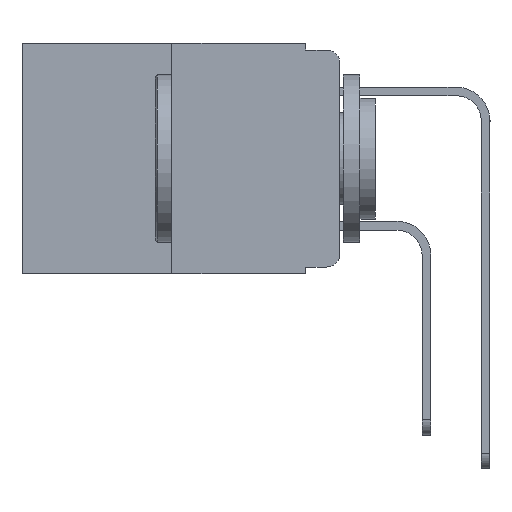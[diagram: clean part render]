
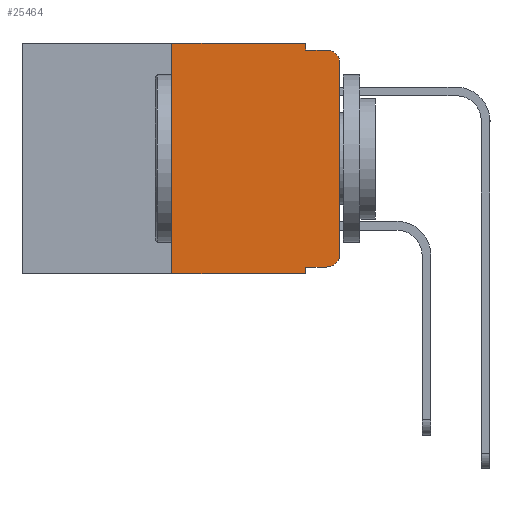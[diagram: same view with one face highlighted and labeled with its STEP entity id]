
A CAD part, left-side view. The second image highlights one B-rep face of the part: STEP entity #25464.
In plain terms, the highlighted planar face has unit normal (-1, 0, 0).
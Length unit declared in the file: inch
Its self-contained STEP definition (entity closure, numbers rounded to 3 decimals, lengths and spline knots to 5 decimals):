
#24 = ORIENTED_EDGE ( 'NONE', *, *, #26438, .T. ) ;
#459 = LINE ( 'NONE', #10308, #4694 ) ;
#638 = CARTESIAN_POINT ( 'NONE',  ( 0., 0.25, 0. ) ) ;
#872 = DIRECTION ( 'NONE',  ( -1., 0., 0. ) ) ;
#988 = CARTESIAN_POINT ( 'NONE',  ( 0., 0., -0.313 ) ) ;
#1020 = CARTESIAN_POINT ( 'NONE',  ( 0., 0.473, 0. ) ) ;
#1045 = VECTOR ( 'NONE', #23767, 39.37008 ) ;
#1234 = VERTEX_POINT ( 'NONE', #17863 ) ;
#1333 = EDGE_CURVE ( 'NONE', #17584, #11940, #21363, .T. ) ;
#1500 = VERTEX_POINT ( 'NONE', #988 ) ;
#1569 = ORIENTED_EDGE ( 'NONE', *, *, #6924, .F. ) ;
#1661 = ORIENTED_EDGE ( 'NONE', *, *, #5514, .F. ) ;
#1730 = DIRECTION ( 'NONE',  ( 0., 0., -1. ) ) ;
#3097 = DIRECTION ( 'NONE',  ( 0., 0., 1. ) ) ;
#3504 = CIRCLE ( 'NONE', #10316, 0.02 ) ;
#4107 = DIRECTION ( 'NONE',  ( 0., -1., 0. ) ) ;
#4131 = EDGE_CURVE ( 'NONE', #1234, #20670, #12058, .T. ) ;
#4135 = CARTESIAN_POINT ( 'NONE',  ( 0., 0.051, -0.01 ) ) ;
#4596 = ORIENTED_EDGE ( 'NONE', *, *, #8318, .T. ) ;
#4694 = VECTOR ( 'NONE', #23948, 39.37008 ) ;
#4937 = CARTESIAN_POINT ( 'NONE',  ( 0., 0., -0.03 ) ) ;
#5241 = CARTESIAN_POINT ( 'NONE',  ( 0., 0.25, 0. ) ) ;
#5342 = FACE_OUTER_BOUND ( 'NONE', #8882, .T. ) ;
#5514 = EDGE_CURVE ( 'NONE', #20888, #10586, #6510, .T. ) ;
#5902 = ORIENTED_EDGE ( 'NONE', *, *, #23820, .T. ) ;
#6167 = PLANE ( 'NONE',  #19599 ) ;
#6510 = LINE ( 'NONE', #13125, #22147 ) ;
#6924 = EDGE_CURVE ( 'NONE', #10586, #23219, #25503, .T. ) ;
#7121 = VERTEX_POINT ( 'NONE', #4937 ) ;
#7140 = DIRECTION ( 'NONE',  ( 0., -1., 0. ) ) ;
#8240 = DIRECTION ( 'NONE',  ( 0., 0., -1. ) ) ;
#8318 = EDGE_CURVE ( 'NONE', #7121, #23219, #20580, .T. ) ;
#8343 = VECTOR ( 'NONE', #18704, 39.37008 ) ;
#8415 = VECTOR ( 'NONE', #3097, 39.37008 ) ;
#8749 = LINE ( 'NONE', #1020, #24350 ) ;
#8882 = EDGE_LOOP ( 'NONE', ( #9433, #4596, #1569, #1661, #17804, #15344, #12168, #11025, #24, #5902 ) ) ;
#8999 = EDGE_CURVE ( 'NONE', #20670, #20888, #8749, .T. ) ;
#9433 = ORIENTED_EDGE ( 'NONE', *, *, #9685, .T. ) ;
#9613 = LINE ( 'NONE', #16665, #8343 ) ;
#9685 = EDGE_CURVE ( 'NONE', #1500, #7121, #13895, .T. ) ;
#9777 = CARTESIAN_POINT ( 'NONE',  ( 0., 0.02, -0.313 ) ) ;
#9812 = CARTESIAN_POINT ( 'NONE',  ( 0., 0.02, -0.01 ) ) ;
#9957 = CARTESIAN_POINT ( 'NONE',  ( 0., 0.051, -0.01 ) ) ;
#9986 = VECTOR ( 'NONE', #4107, 39.37008 ) ;
#10217 = CARTESIAN_POINT ( 'NONE',  ( 0., 0.473, 0. ) ) ;
#10308 = CARTESIAN_POINT ( 'NONE',  ( 0., 0.473, -0.343 ) ) ;
#10316 = AXIS2_PLACEMENT_3D ( 'NONE', #9777, #24016, #11842 ) ;
#10586 = VERTEX_POINT ( 'NONE', #9957 ) ;
#11000 = CARTESIAN_POINT ( 'NONE',  ( 0., 0.051, -0.333 ) ) ;
#11025 = ORIENTED_EDGE ( 'NONE', *, *, #1333, .F. ) ;
#11171 = DIRECTION ( 'NONE',  ( 0., 0., -1. ) ) ;
#11842 = DIRECTION ( 'NONE',  ( 0., 0., -1. ) ) ;
#11940 = VERTEX_POINT ( 'NONE', #12502 ) ;
#12058 = LINE ( 'NONE', #638, #1045 ) ;
#12168 = ORIENTED_EDGE ( 'NONE', *, *, #25477, .T. ) ;
#12502 = CARTESIAN_POINT ( 'NONE',  ( 0., 0.051, -0.343 ) ) ;
#13125 = CARTESIAN_POINT ( 'NONE',  ( 0., 0.051, 0. ) ) ;
#13294 = CARTESIAN_POINT ( 'NONE',  ( 0., 0.02, -0.03 ) ) ;
#13895 = LINE ( 'NONE', #15472, #8415 ) ;
#15100 = AXIS2_PLACEMENT_3D ( 'NONE', #13294, #872, #15342 ) ;
#15298 = VERTEX_POINT ( 'NONE', #23683 ) ;
#15342 = DIRECTION ( 'NONE',  ( 0., 0., -1. ) ) ;
#15344 = ORIENTED_EDGE ( 'NONE', *, *, #4131, .F. ) ;
#15472 = CARTESIAN_POINT ( 'NONE',  ( 0., 0., 0. ) ) ;
#16044 = VECTOR ( 'NONE', #1730, 39.37008 ) ;
#16665 = CARTESIAN_POINT ( 'NONE',  ( 0., 0.051, -0.333 ) ) ;
#17584 = VERTEX_POINT ( 'NONE', #11000 ) ;
#17804 = ORIENTED_EDGE ( 'NONE', *, *, #8999, .F. ) ;
#17863 = CARTESIAN_POINT ( 'NONE',  ( 0., 0.25, -0.343 ) ) ;
#18704 = DIRECTION ( 'NONE',  ( 0., -1., 0. ) ) ;
#18725 = CARTESIAN_POINT ( 'NONE',  ( 0., 0.051, 0. ) ) ;
#19599 = AXIS2_PLACEMENT_3D ( 'NONE', #10217, #20439, #8240 ) ;
#20439 = DIRECTION ( 'NONE',  ( 1., 0., 0. ) ) ;
#20580 = CIRCLE ( 'NONE', #15100, 0.02 ) ;
#20670 = VERTEX_POINT ( 'NONE', #5241 ) ;
#20888 = VERTEX_POINT ( 'NONE', #18725 ) ;
#21363 = LINE ( 'NONE', #23724, #16044 ) ;
#22147 = VECTOR ( 'NONE', #11171, 39.37008 ) ;
#23219 = VERTEX_POINT ( 'NONE', #9812 ) ;
#23683 = CARTESIAN_POINT ( 'NONE',  ( 0., 0.02, -0.333 ) ) ;
#23724 = CARTESIAN_POINT ( 'NONE',  ( 0., 0.051, 0. ) ) ;
#23767 = DIRECTION ( 'NONE',  ( 0., 0., 1. ) ) ;
#23820 = EDGE_CURVE ( 'NONE', #15298, #1500, #3504, .T. ) ;
#23948 = DIRECTION ( 'NONE',  ( 0., -1., 0. ) ) ;
#24016 = DIRECTION ( 'NONE',  ( -1., 0., 0. ) ) ;
#24350 = VECTOR ( 'NONE', #7140, 39.37008 ) ;
#25464 = ADVANCED_FACE ( 'NONE', ( #5342 ), #6167, .F. ) ;
#25477 = EDGE_CURVE ( 'NONE', #1234, #11940, #459, .T. ) ;
#25503 = LINE ( 'NONE', #4135, #9986 ) ;
#26438 = EDGE_CURVE ( 'NONE', #17584, #15298, #9613, .T. ) ;
